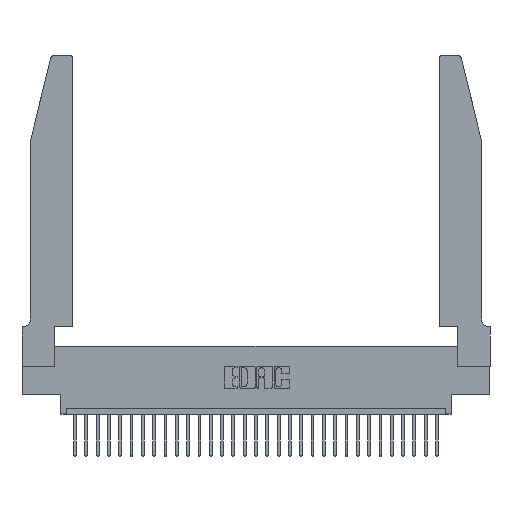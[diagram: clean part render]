
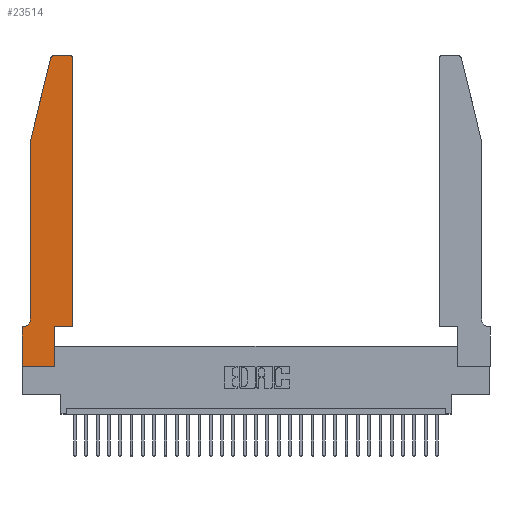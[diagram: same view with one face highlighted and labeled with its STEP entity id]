
A CAD part, top view. The second image highlights one B-rep face of the part: STEP entity #23514.
In plain terms, the highlighted planar face has unit normal (0, 0, 1).
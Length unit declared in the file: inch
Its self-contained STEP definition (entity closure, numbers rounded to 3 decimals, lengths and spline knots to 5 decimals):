
#408 = PLANE ( 'NONE',  #2080 ) ;
#521 = VERTEX_POINT ( 'NONE', #27770 ) ;
#758 = LINE ( 'NONE', #24194, #3399 ) ;
#1041 = VERTEX_POINT ( 'NONE', #11896 ) ;
#1625 = LINE ( 'NONE', #19400, #3498 ) ;
#1695 = ORIENTED_EDGE ( 'NONE', *, *, #3500, .T. ) ;
#2080 = AXIS2_PLACEMENT_3D ( 'NONE', #28845, #15025, #5884 ) ;
#2103 = VERTEX_POINT ( 'NONE', #6226 ) ;
#2697 = CARTESIAN_POINT ( 'NONE',  ( 0.0055, 0.42, 0.37 ) ) ;
#3013 = LINE ( 'NONE', #18610, #23534 ) ;
#3399 = VECTOR ( 'NONE', #27026, 39.37008 ) ;
#3498 = VECTOR ( 'NONE', #28788, 39.37008 ) ;
#3500 = EDGE_CURVE ( 'NONE', #16047, #9999, #3013, .T. ) ;
#4248 = EDGE_CURVE ( 'NONE', #4591, #1041, #29859, .T. ) ;
#4453 = ORIENTED_EDGE ( 'NONE', *, *, #29954, .T. ) ;
#4506 = DIRECTION ( 'NONE',  ( 0., 0., 1. ) ) ;
#4591 = VERTEX_POINT ( 'NONE', #17487 ) ;
#4634 = DIRECTION ( 'NONE',  ( 1., 0., 0. ) ) ;
#4789 = CARTESIAN_POINT ( 'NONE',  ( 0.25487, 2.72718, 0.37 ) ) ;
#4844 = CARTESIAN_POINT ( 'NONE',  ( 0.4505, 0.35, 0.37 ) ) ;
#5043 = CIRCLE ( 'NONE', #7171, 0.03 ) ;
#5154 = VERTEX_POINT ( 'NONE', #25610 ) ;
#5303 = LINE ( 'NONE', #22439, #20986 ) ;
#5884 = DIRECTION ( 'NONE',  ( 1., 0., 0. ) ) ;
#6063 = CARTESIAN_POINT ( 'NONE',  ( 0.284, 2.75, 0.37 ) ) ;
#6226 = CARTESIAN_POINT ( 'NONE',  ( 0.4505, 0.35, 0.37 ) ) ;
#6742 = CARTESIAN_POINT ( 'NONE',  ( 0., 0., 0.37 ) ) ;
#7171 = AXIS2_PLACEMENT_3D ( 'NONE', #9207, #4506, #30462 ) ;
#7187 = CARTESIAN_POINT ( 'NONE',  ( 0.2865, 0., 0.37 ) ) ;
#7459 = AXIS2_PLACEMENT_3D ( 'NONE', #10102, #9901, #14491 ) ;
#7676 = EDGE_CURVE ( 'NONE', #16739, #16047, #5043, .T. ) ;
#7850 = ORIENTED_EDGE ( 'NONE', *, *, #29995, .T. ) ;
#7917 = EDGE_CURVE ( 'NONE', #1041, #16739, #1625, .T. ) ;
#8437 = ORIENTED_EDGE ( 'NONE', *, *, #7676, .T. ) ;
#8505 = DIRECTION ( 'NONE',  ( -1., 0., 0. ) ) ;
#8891 = EDGE_CURVE ( 'NONE', #9999, #16062, #29985, .T. ) ;
#9207 = CARTESIAN_POINT ( 'NONE',  ( 0.284, 2.72, 0.37 ) ) ;
#9650 = EDGE_CURVE ( 'NONE', #521, #28338, #25393, .T. ) ;
#9664 = CARTESIAN_POINT ( 'NONE',  ( 0.2865, 0.35, 0.37 ) ) ;
#9673 = LINE ( 'NONE', #14009, #23072 ) ;
#9703 = CARTESIAN_POINT ( 'NONE',  ( 0.0755, 2., 0.37 ) ) ;
#9783 = CARTESIAN_POINT ( 'NONE',  ( 0.0755, 0.42, 0.37 ) ) ;
#9901 = DIRECTION ( 'NONE',  ( 0., 0., 1. ) ) ;
#9999 = VERTEX_POINT ( 'NONE', #22230 ) ;
#10102 = CARTESIAN_POINT ( 'NONE',  ( 0.4205, 2.72, 0.37 ) ) ;
#10137 = EDGE_CURVE ( 'NONE', #16062, #20641, #12726, .T. ) ;
#10963 = LINE ( 'NONE', #6742, #21017 ) ;
#11800 = EDGE_CURVE ( 'NONE', #2103, #4591, #9673, .T. ) ;
#11896 = CARTESIAN_POINT ( 'NONE',  ( 0.4205, 2.75, 0.37 ) ) ;
#12726 = CIRCLE ( 'NONE', #18912, 0.07 ) ;
#13791 = DIRECTION ( 'NONE',  ( 0., -1., 0. ) ) ;
#13915 = DIRECTION ( 'NONE',  ( 1., 0., 0. ) ) ;
#14009 = CARTESIAN_POINT ( 'NONE',  ( 0.4505, 0.35, 0.37 ) ) ;
#14229 = FACE_OUTER_BOUND ( 'NONE', #24069, .T. ) ;
#14442 = VERTEX_POINT ( 'NONE', #9664 ) ;
#14491 = DIRECTION ( 'NONE',  ( 1., 0., 0. ) ) ;
#14952 = VECTOR ( 'NONE', #13915, 39.37008 ) ;
#15025 = DIRECTION ( 'NONE',  ( 0., 0., 1. ) ) ;
#16047 = VERTEX_POINT ( 'NONE', #4789 ) ;
#16062 = VERTEX_POINT ( 'NONE', #9783 ) ;
#16571 = VECTOR ( 'NONE', #4634, 39.37008 ) ;
#16739 = VERTEX_POINT ( 'NONE', #6063 ) ;
#16755 = CARTESIAN_POINT ( 'NONE',  ( 0., 0., 0.37 ) ) ;
#16758 = ORIENTED_EDGE ( 'NONE', *, *, #8891, .T. ) ;
#17108 = DIRECTION ( 'NONE',  ( -1., 0., 0. ) ) ;
#17180 = ORIENTED_EDGE ( 'NONE', *, *, #11800, .T. ) ;
#17399 = DIRECTION ( 'NONE',  ( 0., 0., -1. ) ) ;
#17487 = CARTESIAN_POINT ( 'NONE',  ( 0.4505, 2.72, 0.37 ) ) ;
#18610 = CARTESIAN_POINT ( 'NONE',  ( 0.0755, 2., 0.37 ) ) ;
#18912 = AXIS2_PLACEMENT_3D ( 'NONE', #2697, #17399, #17108 ) ;
#19018 = DIRECTION ( 'NONE',  ( 0., -1., 0. ) ) ;
#19400 = CARTESIAN_POINT ( 'NONE',  ( 0.2605, 2.75, 0.37 ) ) ;
#20077 = CARTESIAN_POINT ( 'NONE',  ( 0.0055, 0.35, 0.37 ) ) ;
#20641 = VERTEX_POINT ( 'NONE', #20077 ) ;
#20986 = VECTOR ( 'NONE', #8505, 39.37008 ) ;
#21017 = VECTOR ( 'NONE', #13791, 39.37008 ) ;
#22230 = CARTESIAN_POINT ( 'NONE',  ( 0.0755, 2., 0.37 ) ) ;
#22353 = EDGE_CURVE ( 'NONE', #20641, #5154, #5303, .T. ) ;
#22439 = CARTESIAN_POINT ( 'NONE',  ( 0.0755, 0.35, 0.37 ) ) ;
#22547 = EDGE_CURVE ( 'NONE', #28338, #14442, #758, .T. ) ;
#22801 = ORIENTED_EDGE ( 'NONE', *, *, #22547, .T. ) ;
#23072 = VECTOR ( 'NONE', #23280, 39.37008 ) ;
#23280 = DIRECTION ( 'NONE',  ( 0., 1., 0. ) ) ;
#23349 = ORIENTED_EDGE ( 'NONE', *, *, #4248, .T. ) ;
#23443 = DIRECTION ( 'NONE',  ( -0.239, -0.971, 0. ) ) ;
#23514 = ADVANCED_FACE ( 'NONE', ( #14229 ), #408, .T. ) ;
#23534 = VECTOR ( 'NONE', #23443, 39.37008 ) ;
#24069 = EDGE_LOOP ( 'NONE', ( #30800, #8437, #1695, #16758, #26350, #30272, #4453, #27018, #22801, #7850, #17180, #23349 ) ) ;
#24194 = CARTESIAN_POINT ( 'NONE',  ( 0.2865, 0.35, 0.37 ) ) ;
#25393 = LINE ( 'NONE', #16755, #14952 ) ;
#25610 = CARTESIAN_POINT ( 'NONE',  ( 0., 0.35, 0.37 ) ) ;
#26225 = VECTOR ( 'NONE', #19018, 39.37008 ) ;
#26350 = ORIENTED_EDGE ( 'NONE', *, *, #10137, .T. ) ;
#26598 = LINE ( 'NONE', #4844, #16571 ) ;
#27018 = ORIENTED_EDGE ( 'NONE', *, *, #9650, .T. ) ;
#27026 = DIRECTION ( 'NONE',  ( 0., 1., 0. ) ) ;
#27770 = CARTESIAN_POINT ( 'NONE',  ( 0., 0., 0.37 ) ) ;
#28338 = VERTEX_POINT ( 'NONE', #7187 ) ;
#28788 = DIRECTION ( 'NONE',  ( -1., 0., 0. ) ) ;
#28845 = CARTESIAN_POINT ( 'NONE',  ( 0., 0.35, 0.37 ) ) ;
#29859 = CIRCLE ( 'NONE', #7459, 0.03 ) ;
#29954 = EDGE_CURVE ( 'NONE', #5154, #521, #10963, .T. ) ;
#29985 = LINE ( 'NONE', #9703, #26225 ) ;
#29995 = EDGE_CURVE ( 'NONE', #14442, #2103, #26598, .T. ) ;
#30272 = ORIENTED_EDGE ( 'NONE', *, *, #22353, .T. ) ;
#30462 = DIRECTION ( 'NONE',  ( 1., 0., 0. ) ) ;
#30800 = ORIENTED_EDGE ( 'NONE', *, *, #7917, .T. ) ;
